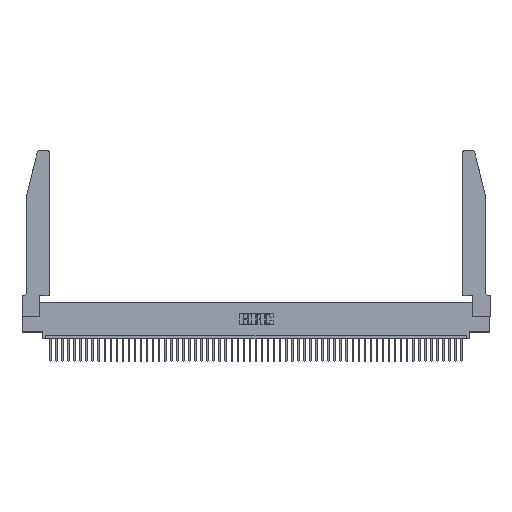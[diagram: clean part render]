
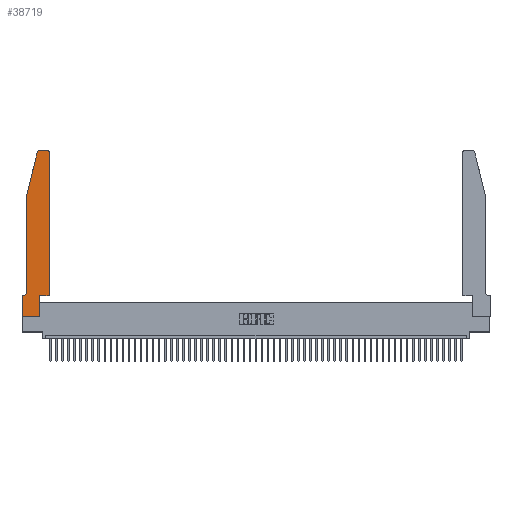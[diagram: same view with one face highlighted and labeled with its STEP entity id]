
A CAD part, top view. The second image highlights one B-rep face of the part: STEP entity #38719.
In plain terms, the highlighted planar face has unit normal (0, 0, 1).
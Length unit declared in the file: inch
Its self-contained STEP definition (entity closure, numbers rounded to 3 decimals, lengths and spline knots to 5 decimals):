
#316 = CARTESIAN_POINT ( 'NONE',  ( 0.4505, 0.35, 0.37 ) ) ;
#598 = LINE ( 'NONE', #12694, #32121 ) ;
#2240 = PLANE ( 'NONE',  #4208 ) ;
#2428 = VERTEX_POINT ( 'NONE', #39788 ) ;
#2593 = VERTEX_POINT ( 'NONE', #18521 ) ;
#3285 = CARTESIAN_POINT ( 'NONE',  ( 0.0755, 0.42, 0.37 ) ) ;
#3313 = VECTOR ( 'NONE', #37736, 39.37008 ) ;
#3472 = DIRECTION ( 'NONE',  ( 0., 1., 0. ) ) ;
#3771 = EDGE_CURVE ( 'NONE', #6403, #15829, #16893, .T. ) ;
#3772 = FACE_OUTER_BOUND ( 'NONE', #33057, .T. ) ;
#4208 = AXIS2_PLACEMENT_3D ( 'NONE', #42673, #14094, #42832 ) ;
#4315 = CARTESIAN_POINT ( 'NONE',  ( 0.0755, 2., 0.37 ) ) ;
#4383 = VECTOR ( 'NONE', #38509, 39.37008 ) ;
#5375 = VECTOR ( 'NONE', #11011, 39.37008 ) ;
#6359 = CARTESIAN_POINT ( 'NONE',  ( 0.4505, 2.72, 0.37 ) ) ;
#6403 = VERTEX_POINT ( 'NONE', #316 ) ;
#6720 = CIRCLE ( 'NONE', #49722, 0.03 ) ;
#6823 = EDGE_CURVE ( 'NONE', #10897, #47398, #8231, .T. ) ;
#6932 = VECTOR ( 'NONE', #52634, 39.37008 ) ;
#8231 = LINE ( 'NONE', #40641, #6932 ) ;
#9571 = CARTESIAN_POINT ( 'NONE',  ( 0.2605, 2.75, 0.37 ) ) ;
#10708 = CARTESIAN_POINT ( 'NONE',  ( 0.4505, 0.35, 0.37 ) ) ;
#10897 = VERTEX_POINT ( 'NONE', #52719 ) ;
#11011 = DIRECTION ( 'NONE',  ( 0., 1., 0. ) ) ;
#11025 = CARTESIAN_POINT ( 'NONE',  ( 0.4205, 2.75, 0.37 ) ) ;
#11302 = CARTESIAN_POINT ( 'NONE',  ( 0., 0., 0.37 ) ) ;
#12274 = DIRECTION ( 'NONE',  ( 1., 0., 0. ) ) ;
#12694 = CARTESIAN_POINT ( 'NONE',  ( 0., 0., 0.37 ) ) ;
#12888 = EDGE_CURVE ( 'NONE', #15829, #51222, #6720, .T. ) ;
#13286 = EDGE_CURVE ( 'NONE', #30070, #16600, #31143, .T. ) ;
#14094 = DIRECTION ( 'NONE',  ( 0., 0., 1. ) ) ;
#14465 = ORIENTED_EDGE ( 'NONE', *, *, #39022, .T. ) ;
#14527 = ORIENTED_EDGE ( 'NONE', *, *, #6823, .T. ) ;
#14631 = CARTESIAN_POINT ( 'NONE',  ( 0., 0., 0.37 ) ) ;
#14953 = ORIENTED_EDGE ( 'NONE', *, *, #23246, .T. ) ;
#15528 = EDGE_CURVE ( 'NONE', #50490, #26611, #598, .T. ) ;
#15829 = VERTEX_POINT ( 'NONE', #6359 ) ;
#16600 = VERTEX_POINT ( 'NONE', #51296 ) ;
#16893 = LINE ( 'NONE', #28143, #52854 ) ;
#17448 = LINE ( 'NONE', #4315, #3313 ) ;
#18521 = CARTESIAN_POINT ( 'NONE',  ( 0.284, 2.75, 0.37 ) ) ;
#20393 = CARTESIAN_POINT ( 'NONE',  ( 0.284, 2.72, 0.37 ) ) ;
#20757 = VERTEX_POINT ( 'NONE', #25916 ) ;
#22591 = DIRECTION ( 'NONE',  ( 1., 0., 0. ) ) ;
#23246 = EDGE_CURVE ( 'NONE', #20757, #10897, #17448, .T. ) ;
#25349 = EDGE_CURVE ( 'NONE', #16600, #6403, #30104, .T. ) ;
#25916 = CARTESIAN_POINT ( 'NONE',  ( 0.25487, 2.72718, 0.37 ) ) ;
#26611 = VERTEX_POINT ( 'NONE', #11302 ) ;
#26615 = LINE ( 'NONE', #37998, #33000 ) ;
#26984 = CARTESIAN_POINT ( 'NONE',  ( 0.2865, 0., 0.37 ) ) ;
#27002 = CARTESIAN_POINT ( 'NONE',  ( 0.0055, 0.42, 0.37 ) ) ;
#28143 = CARTESIAN_POINT ( 'NONE',  ( 0.4505, 0.35, 0.37 ) ) ;
#29538 = EDGE_CURVE ( 'NONE', #51222, #2593, #48077, .T. ) ;
#30070 = VERTEX_POINT ( 'NONE', #26984 ) ;
#30103 = ORIENTED_EDGE ( 'NONE', *, *, #3771, .T. ) ;
#30104 = LINE ( 'NONE', #10708, #32027 ) ;
#30369 = CARTESIAN_POINT ( 'NONE',  ( 0., 0.35, 0.37 ) ) ;
#30924 = DIRECTION ( 'NONE',  ( 0., 0., -1. ) ) ;
#31143 = LINE ( 'NONE', #47815, #5375 ) ;
#31697 = VECTOR ( 'NONE', #22591, 39.37008 ) ;
#31766 = ORIENTED_EDGE ( 'NONE', *, *, #47034, .T. ) ;
#32027 = VECTOR ( 'NONE', #48216, 39.37008 ) ;
#32121 = VECTOR ( 'NONE', #33582, 39.37008 ) ;
#33000 = VECTOR ( 'NONE', #42130, 39.37008 ) ;
#33057 = EDGE_LOOP ( 'NONE', ( #41678, #14465, #14953, #14527, #34571, #31766, #40317, #40649, #36395, #35305, #30103, #46985 ) ) ;
#33582 = DIRECTION ( 'NONE',  ( 0., -1., 0. ) ) ;
#34571 = ORIENTED_EDGE ( 'NONE', *, *, #37553, .T. ) ;
#35305 = ORIENTED_EDGE ( 'NONE', *, *, #25349, .T. ) ;
#35550 = LINE ( 'NONE', #14631, #31697 ) ;
#36395 = ORIENTED_EDGE ( 'NONE', *, *, #13286, .T. ) ;
#37553 = EDGE_CURVE ( 'NONE', #47398, #2428, #44993, .T. ) ;
#37736 = DIRECTION ( 'NONE',  ( -0.239, -0.971, 0. ) ) ;
#37819 = DIRECTION ( 'NONE',  ( 1., 0., 0. ) ) ;
#37998 = CARTESIAN_POINT ( 'NONE',  ( 0.0755, 0.35, 0.37 ) ) ;
#38172 = DIRECTION ( 'NONE',  ( 0., 0., 1. ) ) ;
#38509 = DIRECTION ( 'NONE',  ( -1., 0., 0. ) ) ;
#38719 = ADVANCED_FACE ( 'NONE', ( #3772 ), #2240, .T. ) ;
#39022 = EDGE_CURVE ( 'NONE', #2593, #20757, #43345, .T. ) ;
#39788 = CARTESIAN_POINT ( 'NONE',  ( 0.0055, 0.35, 0.37 ) ) ;
#40317 = ORIENTED_EDGE ( 'NONE', *, *, #15528, .T. ) ;
#40641 = CARTESIAN_POINT ( 'NONE',  ( 0.0755, 2., 0.37 ) ) ;
#40649 = ORIENTED_EDGE ( 'NONE', *, *, #51269, .T. ) ;
#41678 = ORIENTED_EDGE ( 'NONE', *, *, #29538, .T. ) ;
#42130 = DIRECTION ( 'NONE',  ( -1., 0., 0. ) ) ;
#42308 = CARTESIAN_POINT ( 'NONE',  ( 0.4205, 2.72, 0.37 ) ) ;
#42384 = AXIS2_PLACEMENT_3D ( 'NONE', #27002, #30924, #47393 ) ;
#42673 = CARTESIAN_POINT ( 'NONE',  ( 0., 0.35, 0.37 ) ) ;
#42832 = DIRECTION ( 'NONE',  ( 1., 0., 0. ) ) ;
#43345 = CIRCLE ( 'NONE', #43771, 0.03 ) ;
#43771 = AXIS2_PLACEMENT_3D ( 'NONE', #20393, #49086, #12274 ) ;
#44993 = CIRCLE ( 'NONE', #42384, 0.07 ) ;
#46985 = ORIENTED_EDGE ( 'NONE', *, *, #12888, .T. ) ;
#47034 = EDGE_CURVE ( 'NONE', #2428, #50490, #26615, .T. ) ;
#47393 = DIRECTION ( 'NONE',  ( -1., 0., 0. ) ) ;
#47398 = VERTEX_POINT ( 'NONE', #3285 ) ;
#47815 = CARTESIAN_POINT ( 'NONE',  ( 0.2865, 0.35, 0.37 ) ) ;
#48077 = LINE ( 'NONE', #9571, #4383 ) ;
#48216 = DIRECTION ( 'NONE',  ( 1., 0., 0. ) ) ;
#49086 = DIRECTION ( 'NONE',  ( 0., 0., 1. ) ) ;
#49722 = AXIS2_PLACEMENT_3D ( 'NONE', #42308, #38172, #37819 ) ;
#50490 = VERTEX_POINT ( 'NONE', #30369 ) ;
#51222 = VERTEX_POINT ( 'NONE', #11025 ) ;
#51269 = EDGE_CURVE ( 'NONE', #26611, #30070, #35550, .T. ) ;
#51296 = CARTESIAN_POINT ( 'NONE',  ( 0.2865, 0.35, 0.37 ) ) ;
#52634 = DIRECTION ( 'NONE',  ( 0., -1., 0. ) ) ;
#52719 = CARTESIAN_POINT ( 'NONE',  ( 0.0755, 2., 0.37 ) ) ;
#52854 = VECTOR ( 'NONE', #3472, 39.37008 ) ;
